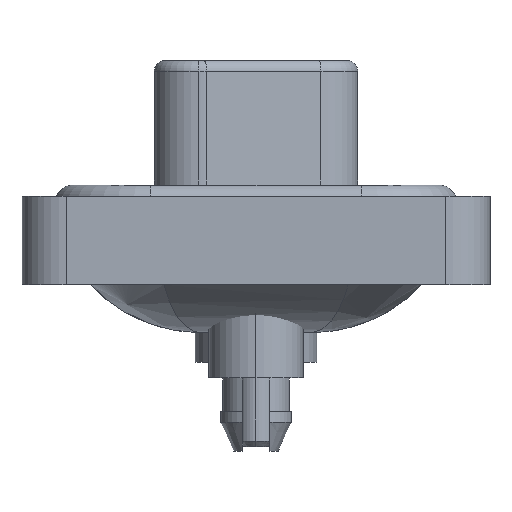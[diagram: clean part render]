
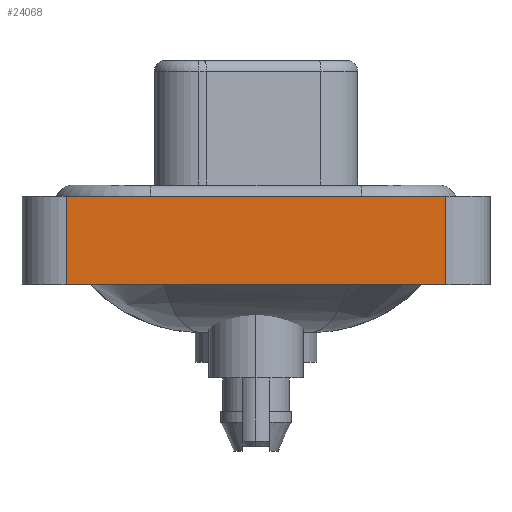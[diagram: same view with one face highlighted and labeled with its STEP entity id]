
A CAD part, left-side view. The second image highlights one B-rep face of the part: STEP entity #24068.
In plain terms, the highlighted planar face has unit normal (-1, 0, 0).
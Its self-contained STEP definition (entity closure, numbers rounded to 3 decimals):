
#408 = AXIS2_PLACEMENT_3D ( 'NONE', #10150, #4639, #19469 ) ;
#793 = EDGE_CURVE ( 'NONE', #21002, #16661, #15164, .T. ) ;
#1582 = DIRECTION ( 'NONE',  ( 0., 0., 1. ) ) ;
#1860 = CARTESIAN_POINT ( 'NONE',  ( -7.3, -8.55, -3.6 ) ) ;
#3424 = LINE ( 'NONE', #9155, #4933 ) ;
#4141 = CARTESIAN_POINT ( 'NONE',  ( -7.3, -8.55, 0.4 ) ) ;
#4175 = DIRECTION ( 'NONE',  ( 0., 0., 1. ) ) ;
#4639 = DIRECTION ( 'NONE',  ( -1., 0., 0. ) ) ;
#4933 = VECTOR ( 'NONE', #1582, 1000. ) ;
#5866 = EDGE_CURVE ( 'NONE', #22794, #16661, #24106, .T. ) ;
#6264 = ORIENTED_EDGE ( 'NONE', *, *, #23819, .T. ) ;
#9033 = DIRECTION ( 'NONE',  ( 0., -1., 0. ) ) ;
#9155 = CARTESIAN_POINT ( 'NONE',  ( -7.3, 8.55, -3.6 ) ) ;
#10150 = CARTESIAN_POINT ( 'NONE',  ( -7.3, -8.55, -3.6 ) ) ;
#11702 = VERTEX_POINT ( 'NONE', #23828 ) ;
#11774 = CARTESIAN_POINT ( 'NONE',  ( -7.3, -8.55, 0.4 ) ) ;
#11966 = ORIENTED_EDGE ( 'NONE', *, *, #20209, .F. ) ;
#12001 = PLANE ( 'NONE',  #408 ) ;
#13325 = DIRECTION ( 'NONE',  ( 0., -1., 0. ) ) ;
#14814 = LINE ( 'NONE', #22020, #19057 ) ;
#15164 = LINE ( 'NONE', #4141, #21175 ) ;
#16661 = VERTEX_POINT ( 'NONE', #11774 ) ;
#16722 = ORIENTED_EDGE ( 'NONE', *, *, #5866, .T. ) ;
#17010 = VECTOR ( 'NONE', #4175, 1000. ) ;
#17744 = FACE_OUTER_BOUND ( 'NONE', #23377, .T. ) ;
#17895 = CARTESIAN_POINT ( 'NONE',  ( -7.3, -8.55, -3.6 ) ) ;
#18182 = CARTESIAN_POINT ( 'NONE',  ( -7.3, 8.55, 0.4 ) ) ;
#19057 = VECTOR ( 'NONE', #9033, 1000. ) ;
#19469 = DIRECTION ( 'NONE',  ( 0., 0., 1. ) ) ;
#20209 = EDGE_CURVE ( 'NONE', #11702, #21002, #3424, .T. ) ;
#21002 = VERTEX_POINT ( 'NONE', #18182 ) ;
#21175 = VECTOR ( 'NONE', #13325, 1000. ) ;
#21185 = ORIENTED_EDGE ( 'NONE', *, *, #793, .F. ) ;
#22020 = CARTESIAN_POINT ( 'NONE',  ( -7.3, -8.55, -3.6 ) ) ;
#22794 = VERTEX_POINT ( 'NONE', #17895 ) ;
#23377 = EDGE_LOOP ( 'NONE', ( #16722, #21185, #11966, #6264 ) ) ;
#23819 = EDGE_CURVE ( 'NONE', #11702, #22794, #14814, .T. ) ;
#23828 = CARTESIAN_POINT ( 'NONE',  ( -7.3, 8.55, -3.6 ) ) ;
#24068 = ADVANCED_FACE ( 'NONE', ( #17744 ), #12001, .T. ) ;
#24106 = LINE ( 'NONE', #1860, #17010 ) ;
